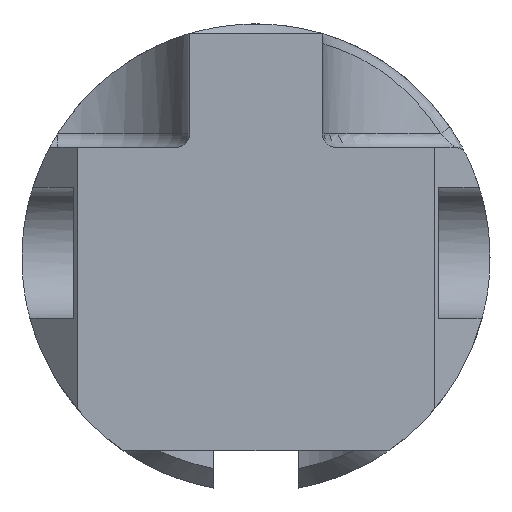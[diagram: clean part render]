
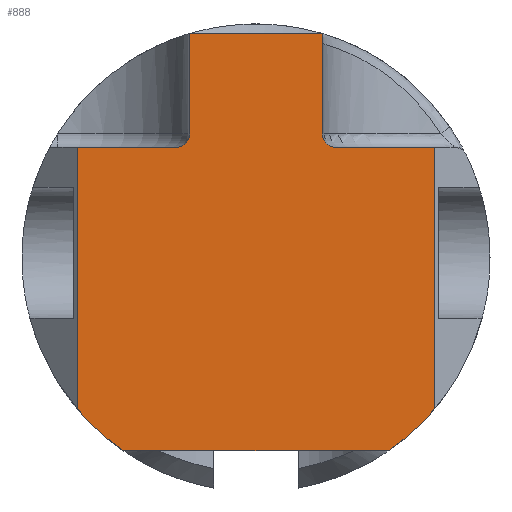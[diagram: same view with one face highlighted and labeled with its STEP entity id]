
A CAD part, front view. The second image highlights one B-rep face of the part: STEP entity #888.
In plain terms, the highlighted planar face has unit normal (0, -1, 0).
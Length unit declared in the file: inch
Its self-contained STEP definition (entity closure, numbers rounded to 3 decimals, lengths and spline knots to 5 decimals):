
#50=CIRCLE('',#957,0.4375);
#51=CIRCLE('',#958,0.4375);
#52=CIRCLE('',#959,0.025);
#53=CIRCLE('',#960,0.025);
#90=FACE_OUTER_BOUND('',#138,.T.);
#138=EDGE_LOOP('',(#700,#701,#702,#703,#704,#705,#706,#707,#708,#709,#710,
#711));
#232=LINE('',#1853,#303);
#239=LINE('',#1874,#310);
#245=LINE('',#1888,#316);
#246=LINE('',#1891,#317);
#247=LINE('',#1895,#318);
#248=LINE('',#1897,#319);
#249=LINE('',#1899,#320);
#250=LINE('',#1902,#321);
#303=VECTOR('',#1075,0.3937);
#310=VECTOR('',#1090,0.3937);
#316=VECTOR('',#1106,0.3937);
#317=VECTOR('',#1109,0.3937);
#318=VECTOR('',#1112,0.3937);
#319=VECTOR('',#1113,0.3937);
#320=VECTOR('',#1114,0.3937);
#321=VECTOR('',#1117,0.3937);
#393=VERTEX_POINT('',#1850);
#394=VERTEX_POINT('',#1852);
#403=VERTEX_POINT('',#1871);
#404=VERTEX_POINT('',#1873);
#406=VERTEX_POINT('',#1885);
#407=VERTEX_POINT('',#1887);
#408=VERTEX_POINT('',#1890);
#409=VERTEX_POINT('',#1892);
#410=VERTEX_POINT('',#1894);
#411=VERTEX_POINT('',#1896);
#412=VERTEX_POINT('',#1898);
#413=VERTEX_POINT('',#1900);
#501=EDGE_CURVE('',#394,#393,#232,.T.);
#511=EDGE_CURVE('',#404,#403,#239,.T.);
#518=EDGE_CURVE('',#406,#393,#50,.T.);
#519=EDGE_CURVE('',#406,#407,#245,.T.);
#520=EDGE_CURVE('',#404,#407,#51,.T.);
#521=EDGE_CURVE('',#403,#408,#246,.T.);
#522=EDGE_CURVE('',#409,#408,#52,.T.);
#523=EDGE_CURVE('',#409,#410,#247,.T.);
#524=EDGE_CURVE('',#411,#410,#248,.T.);
#525=EDGE_CURVE('',#411,#412,#249,.T.);
#526=EDGE_CURVE('',#413,#412,#53,.T.);
#527=EDGE_CURVE('',#413,#394,#250,.T.);
#700=ORIENTED_EDGE('',*,*,#501,.T.);
#701=ORIENTED_EDGE('',*,*,#518,.F.);
#702=ORIENTED_EDGE('',*,*,#519,.T.);
#703=ORIENTED_EDGE('',*,*,#520,.F.);
#704=ORIENTED_EDGE('',*,*,#511,.T.);
#705=ORIENTED_EDGE('',*,*,#521,.T.);
#706=ORIENTED_EDGE('',*,*,#522,.F.);
#707=ORIENTED_EDGE('',*,*,#523,.T.);
#708=ORIENTED_EDGE('',*,*,#524,.F.);
#709=ORIENTED_EDGE('',*,*,#525,.T.);
#710=ORIENTED_EDGE('',*,*,#526,.F.);
#711=ORIENTED_EDGE('',*,*,#527,.T.);
#851=PLANE('',#956);
#888=ADVANCED_FACE('',(#90),#851,.F.);
#956=AXIS2_PLACEMENT_3D('',#1884,#1102,#1103);
#957=AXIS2_PLACEMENT_3D('',#1886,#1104,#1105);
#958=AXIS2_PLACEMENT_3D('',#1889,#1107,#1108);
#959=AXIS2_PLACEMENT_3D('',#1893,#1110,#1111);
#960=AXIS2_PLACEMENT_3D('',#1901,#1115,#1116);
#1075=DIRECTION('',(0.,0.,-1.));
#1090=DIRECTION('',(0.,0.,1.));
#1102=DIRECTION('center_axis',(0.,1.,0.));
#1103=DIRECTION('ref_axis',(1.,0.,0.));
#1104=DIRECTION('center_axis',(0.,1.,0.));
#1105=DIRECTION('ref_axis',(1.,0.,0.));
#1106=DIRECTION('',(1.,0.,0.));
#1107=DIRECTION('center_axis',(0.,1.,0.));
#1108=DIRECTION('ref_axis',(1.,0.,0.));
#1109=DIRECTION('',(-1.,0.,0.));
#1110=DIRECTION('center_axis',(0.,-1.,0.));
#1111=DIRECTION('ref_axis',(-0.707,0.,-0.707));
#1112=DIRECTION('',(0.,0.,1.));
#1113=DIRECTION('',(1.,0.,0.));
#1114=DIRECTION('',(0.,0.,-1.));
#1115=DIRECTION('center_axis',(0.,-1.,0.));
#1116=DIRECTION('ref_axis',(0.707,0.,-0.707));
#1117=DIRECTION('',(-1.,0.,0.));
#1850=CARTESIAN_POINT('',(-0.3342,0.,-0.28235));
#1852=CARTESIAN_POINT('',(-0.3342,0.,0.20674));
#1853=CARTESIAN_POINT('',(-0.3342,0.,0.0147));
#1871=CARTESIAN_POINT('',(0.3342,0.,0.20674));
#1873=CARTESIAN_POINT('',(0.3342,0.,-0.28235));
#1874=CARTESIAN_POINT('',(0.3342,0.,0.0147));
#1884=CARTESIAN_POINT('Origin',(0.,0.,0.0294));
#1885=CARTESIAN_POINT('',(-0.2475,0.,-0.36076));
#1886=CARTESIAN_POINT('Origin',(0.,0.,0.));
#1887=CARTESIAN_POINT('',(0.2475,0.,-0.36076));
#1888=CARTESIAN_POINT('',(0.,0.,-0.36076));
#1889=CARTESIAN_POINT('Origin',(0.,0.,0.));
#1890=CARTESIAN_POINT('',(0.149,0.,0.20674));
#1891=CARTESIAN_POINT('',(0.19279,0.,0.20674));
#1892=CARTESIAN_POINT('',(0.124,0.,0.23174));
#1893=CARTESIAN_POINT('Origin',(0.149,0.,0.23174));
#1894=CARTESIAN_POINT('',(0.124,0.,0.41956));
#1895=CARTESIAN_POINT('',(0.124,0.,0.11807));
#1896=CARTESIAN_POINT('',(-0.124,0.,0.41956));
#1897=CARTESIAN_POINT('',(-0.124,0.,0.41956));
#1898=CARTESIAN_POINT('',(-0.124,0.,0.23174));
#1899=CARTESIAN_POINT('',(-0.124,0.,0.22448));
#1900=CARTESIAN_POINT('',(-0.149,0.,0.20674));
#1901=CARTESIAN_POINT('Origin',(-0.149,0.,0.23174));
#1902=CARTESIAN_POINT('',(-0.062,0.,0.20674));
